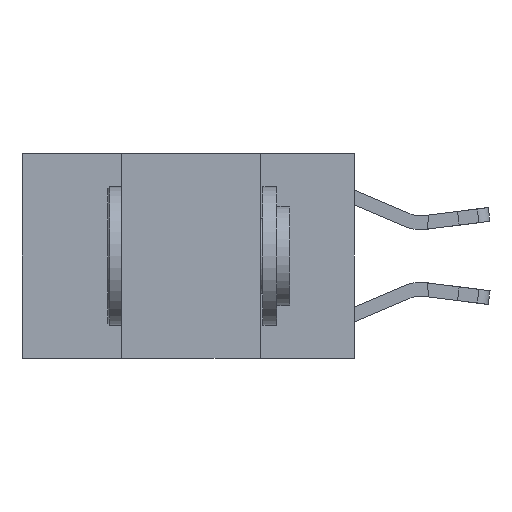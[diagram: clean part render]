
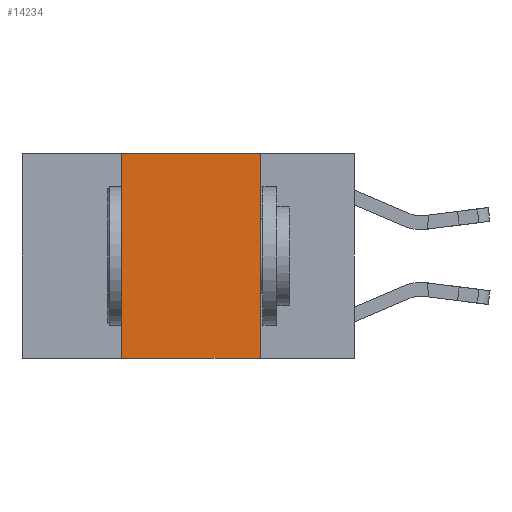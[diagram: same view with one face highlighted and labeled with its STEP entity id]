
A CAD part, left-side view. The second image highlights one B-rep face of the part: STEP entity #14234.
In plain terms, the highlighted planar face has unit normal (-1, 0, 0).
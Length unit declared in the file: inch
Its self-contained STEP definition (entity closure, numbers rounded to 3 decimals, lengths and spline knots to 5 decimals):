
#1027 = LINE ( 'NONE', #3724, #5609 ) ;
#2259 = LINE ( 'NONE', #13267, #10806 ) ;
#3724 = CARTESIAN_POINT ( 'NONE',  ( 0., 0.6, 0. ) ) ;
#5609 = VECTOR ( 'NONE', #5637, 39.37008 ) ;
#5637 = DIRECTION ( 'NONE',  ( 0., -1., 0. ) ) ;
#7085 = VECTOR ( 'NONE', #21718, 39.37008 ) ;
#7103 = CARTESIAN_POINT ( 'NONE',  ( 0., 0.17, 0. ) ) ;
#9093 = PLANE ( 'NONE',  #10132 ) ;
#10132 = AXIS2_PLACEMENT_3D ( 'NONE', #24265, #11063, #24343 ) ;
#10806 = VECTOR ( 'NONE', #24628, 39.37008 ) ;
#10933 = VERTEX_POINT ( 'NONE', #20816 ) ;
#11063 = DIRECTION ( 'NONE',  ( 1., 0., 0. ) ) ;
#11805 = DIRECTION ( 'NONE',  ( 0., 0., 1. ) ) ;
#13267 = CARTESIAN_POINT ( 'NONE',  ( 0., 0.17, 0. ) ) ;
#13814 = LINE ( 'NONE', #21264, #23326 ) ;
#13963 = EDGE_CURVE ( 'NONE', #18375, #17659, #22374, .T. ) ;
#14234 = ADVANCED_FACE ( 'NONE', ( #23588 ), #9093, .F. ) ;
#14389 = CARTESIAN_POINT ( 'NONE',  ( 0., 0.17, -0.37 ) ) ;
#17659 = VERTEX_POINT ( 'NONE', #14389 ) ;
#17839 = VERTEX_POINT ( 'NONE', #7103 ) ;
#18331 = ORIENTED_EDGE ( 'NONE', *, *, #13963, .T. ) ;
#18375 = VERTEX_POINT ( 'NONE', #23070 ) ;
#19059 = EDGE_CURVE ( 'NONE', #18375, #10933, #13814, .T. ) ;
#19828 = CARTESIAN_POINT ( 'NONE',  ( 0., 0.6, -0.37 ) ) ;
#20352 = EDGE_CURVE ( 'NONE', #17839, #17659, #2259, .T. ) ;
#20384 = EDGE_CURVE ( 'NONE', #10933, #17839, #1027, .T. ) ;
#20816 = CARTESIAN_POINT ( 'NONE',  ( 0., 0.42, 0. ) ) ;
#21264 = CARTESIAN_POINT ( 'NONE',  ( 0., 0.42, 0. ) ) ;
#21718 = DIRECTION ( 'NONE',  ( 0., -1., 0. ) ) ;
#22374 = LINE ( 'NONE', #19828, #7085 ) ;
#22629 = EDGE_LOOP ( 'NONE', ( #22771, #23087, #24829, #18331 ) ) ;
#22771 = ORIENTED_EDGE ( 'NONE', *, *, #20352, .F. ) ;
#23070 = CARTESIAN_POINT ( 'NONE',  ( 0., 0.42, -0.37 ) ) ;
#23087 = ORIENTED_EDGE ( 'NONE', *, *, #20384, .F. ) ;
#23326 = VECTOR ( 'NONE', #11805, 39.37008 ) ;
#23588 = FACE_OUTER_BOUND ( 'NONE', #22629, .T. ) ;
#24265 = CARTESIAN_POINT ( 'NONE',  ( 0., 0.6, 0. ) ) ;
#24343 = DIRECTION ( 'NONE',  ( 0., 0., -1. ) ) ;
#24628 = DIRECTION ( 'NONE',  ( 0., 0., -1. ) ) ;
#24829 = ORIENTED_EDGE ( 'NONE', *, *, #19059, .F. ) ;
